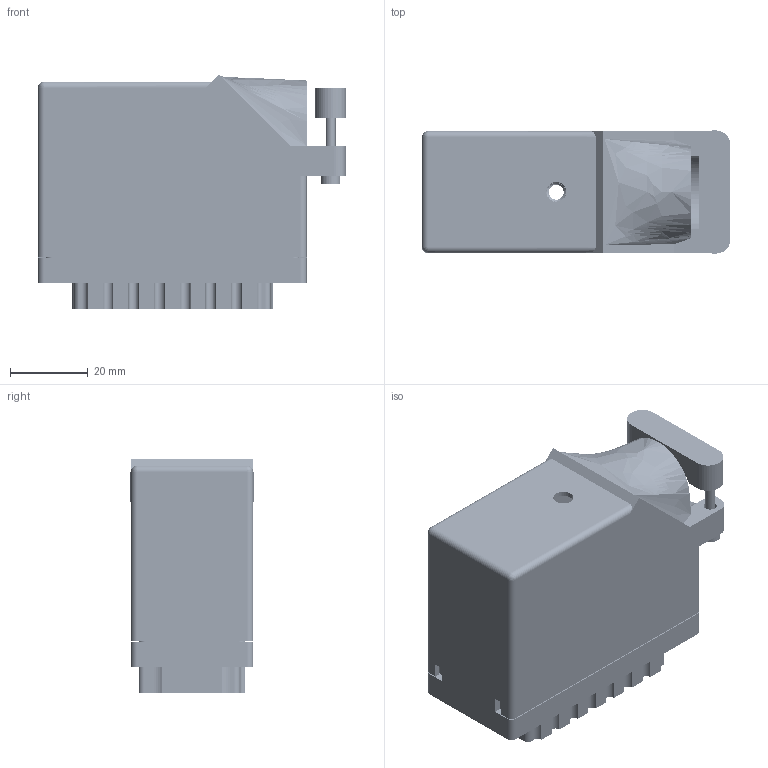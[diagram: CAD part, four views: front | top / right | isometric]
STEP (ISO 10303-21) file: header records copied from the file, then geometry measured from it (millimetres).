
FILE_DESCRIPTION (( 'STEP AP203' ), '1' );
FILE_NAME ('516-090-501-626.STEP', '2020-09-08T18:33:00', ( '' ), ( '' ), 'SwSTEP 2.0', 'SolidWorks 2020', '' );
FILE_SCHEMA (( 'CONFIG_CONTROL_DESIGN' ));
Length unit declared in the file: inch
Products named in the file (5): 516 Part Receptacle_090; 516-292-001_501 Contact; 516-090-501-626; 516-230-001_Plastic - 090 Side Entry; 516-252-095-100
Assembly tree (94 placements, depth 2):
  516-090-501-626
    516 Part Receptacle_090
    516-292-001_501 Contact  x91
    516-230-001_Plastic - 090 Side Entry
    516-252-095-100
Bounding box: 79.2 x 31.75 x 60.37 mm (x, y, z)
Volume: 41013.3 mm3; surface area: 69124.8 mm2
Topology: 94 solids, 94 shells, 8598 faces, 24963 edges, 16575 vertices
Faces by surface type: plane 5154, cylinder 2875, bspline 555, cone 12, sphere 2
Entity records: 76551 total; most frequent: CARTESIAN_POINT 15001, ORIENTED_EDGE 12482, DIRECTION 12147, EDGE_CURVE 6241, VECTOR 4563, LINE 4563, VERTEX_POINT 4155, AXIS2_PLACEMENT_3D 3792
